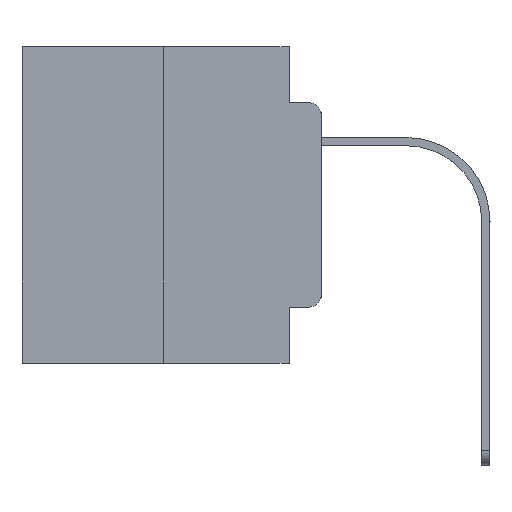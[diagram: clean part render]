
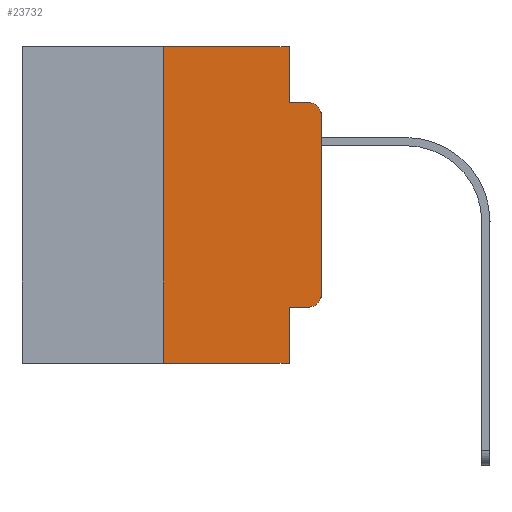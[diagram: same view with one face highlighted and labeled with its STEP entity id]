
A CAD part, left-side view. The second image highlights one B-rep face of the part: STEP entity #23732.
In plain terms, the highlighted planar face has unit normal (-1, 0, 0).
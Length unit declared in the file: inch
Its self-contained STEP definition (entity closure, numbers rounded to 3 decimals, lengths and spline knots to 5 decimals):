
#947 = DIRECTION ( 'NONE',  ( 0., 0., -1. ) ) ;
#1377 = VERTEX_POINT ( 'NONE', #18066 ) ;
#1506 = CARTESIAN_POINT ( 'NONE',  ( 0., 0.25, -0.5 ) ) ;
#1609 = ORIENTED_EDGE ( 'NONE', *, *, #25175, .T. ) ;
#1762 = DIRECTION ( 'NONE',  ( 0., 0., -1. ) ) ;
#2124 = LINE ( 'NONE', #24417, #17803 ) ;
#2192 = EDGE_CURVE ( 'NONE', #19842, #1377, #24350, .T. ) ;
#2422 = EDGE_CURVE ( 'NONE', #10947, #17427, #18857, .T. ) ;
#3428 = EDGE_LOOP ( 'NONE', ( #13011, #10443, #11672, #5072, #9242, #23364, #1609, #8215, #8665, #24004 ) ) ;
#3785 = CARTESIAN_POINT ( 'NONE',  ( 0., 0.02, -0.4115 ) ) ;
#4197 = DIRECTION ( 'NONE',  ( 1., 0., 0. ) ) ;
#4247 = VERTEX_POINT ( 'NONE', #20946 ) ;
#4611 = VERTEX_POINT ( 'NONE', #22001 ) ;
#4989 = EDGE_CURVE ( 'NONE', #5991, #12373, #5500, .T. ) ;
#5072 = ORIENTED_EDGE ( 'NONE', *, *, #4989, .F. ) ;
#5221 = VERTEX_POINT ( 'NONE', #23265 ) ;
#5241 = VECTOR ( 'NONE', #11041, 39.37008 ) ;
#5360 = VECTOR ( 'NONE', #20529, 39.37008 ) ;
#5500 = LINE ( 'NONE', #20105, #22232 ) ;
#5735 = CARTESIAN_POINT ( 'NONE',  ( 0., 0.051, -0.0885 ) ) ;
#5933 = CARTESIAN_POINT ( 'NONE',  ( 0., 0., 0. ) ) ;
#5991 = VERTEX_POINT ( 'NONE', #19231 ) ;
#6164 = DIRECTION ( 'NONE',  ( 0., 0., 1. ) ) ;
#6793 = LINE ( 'NONE', #20867, #22208 ) ;
#7265 = EDGE_CURVE ( 'NONE', #4247, #5991, #6793, .T. ) ;
#7320 = EDGE_CURVE ( 'NONE', #5221, #4611, #13033, .T. ) ;
#8069 = CARTESIAN_POINT ( 'NONE',  ( 0., 0.051, -0.0885 ) ) ;
#8214 = VECTOR ( 'NONE', #14073, 39.37008 ) ;
#8215 = ORIENTED_EDGE ( 'NONE', *, *, #7320, .F. ) ;
#8660 = DIRECTION ( 'NONE',  ( 0., -1., 0. ) ) ;
#8665 = ORIENTED_EDGE ( 'NONE', *, *, #16929, .T. ) ;
#9242 = ORIENTED_EDGE ( 'NONE', *, *, #7265, .F. ) ;
#9701 = VECTOR ( 'NONE', #24666, 39.37008 ) ;
#9929 = AXIS2_PLACEMENT_3D ( 'NONE', #12267, #19970, #1762 ) ;
#10443 = ORIENTED_EDGE ( 'NONE', *, *, #2422, .T. ) ;
#10947 = VERTEX_POINT ( 'NONE', #19371 ) ;
#11041 = DIRECTION ( 'NONE',  ( 0., 0., -1. ) ) ;
#11065 = EDGE_CURVE ( 'NONE', #26241, #4247, #18271, .T. ) ;
#11672 = ORIENTED_EDGE ( 'NONE', *, *, #14029, .F. ) ;
#12267 = CARTESIAN_POINT ( 'NONE',  ( 0., 0.02, -0.3915 ) ) ;
#12313 = DIRECTION ( 'NONE',  ( 0., 0., -1. ) ) ;
#12373 = VERTEX_POINT ( 'NONE', #8069 ) ;
#13011 = ORIENTED_EDGE ( 'NONE', *, *, #23747, .T. ) ;
#13033 = LINE ( 'NONE', #15281, #5241 ) ;
#13389 = VECTOR ( 'NONE', #6164, 39.37008 ) ;
#14029 = EDGE_CURVE ( 'NONE', #12373, #17427, #20067, .T. ) ;
#14073 = DIRECTION ( 'NONE',  ( 0., -1., 0. ) ) ;
#15281 = CARTESIAN_POINT ( 'NONE',  ( 0., 0.051, 0. ) ) ;
#15462 = AXIS2_PLACEMENT_3D ( 'NONE', #23257, #17417, #947 ) ;
#16158 = FACE_OUTER_BOUND ( 'NONE', #3428, .T. ) ;
#16426 = LINE ( 'NONE', #5933, #5360 ) ;
#16591 = CARTESIAN_POINT ( 'NONE',  ( 0., 0.473, -0.5 ) ) ;
#16662 = CARTESIAN_POINT ( 'NONE',  ( 0., 0.25, 0. ) ) ;
#16929 = EDGE_CURVE ( 'NONE', #5221, #19842, #2124, .T. ) ;
#17417 = DIRECTION ( 'NONE',  ( -1., 0., 0. ) ) ;
#17427 = VERTEX_POINT ( 'NONE', #20401 ) ;
#17803 = VECTOR ( 'NONE', #22436, 39.37008 ) ;
#18066 = CARTESIAN_POINT ( 'NONE',  ( 0., 0., -0.3915 ) ) ;
#18271 = LINE ( 'NONE', #16662, #13389 ) ;
#18857 = CIRCLE ( 'NONE', #15462, 0.02 ) ;
#19231 = CARTESIAN_POINT ( 'NONE',  ( 0., 0.051, 0. ) ) ;
#19371 = CARTESIAN_POINT ( 'NONE',  ( 0., 0., -0.1085 ) ) ;
#19842 = VERTEX_POINT ( 'NONE', #3785 ) ;
#19970 = DIRECTION ( 'NONE',  ( -1., 0., 0. ) ) ;
#20067 = LINE ( 'NONE', #5735, #8214 ) ;
#20105 = CARTESIAN_POINT ( 'NONE',  ( 0., 0.051, 0. ) ) ;
#20401 = CARTESIAN_POINT ( 'NONE',  ( 0., 0.02, -0.0885 ) ) ;
#20529 = DIRECTION ( 'NONE',  ( 0., 0., 1. ) ) ;
#20867 = CARTESIAN_POINT ( 'NONE',  ( 0., 0.473, 0. ) ) ;
#20946 = CARTESIAN_POINT ( 'NONE',  ( 0., 0.25, 0. ) ) ;
#20960 = LINE ( 'NONE', #16591, #9701 ) ;
#22001 = CARTESIAN_POINT ( 'NONE',  ( 0., 0.051, -0.5 ) ) ;
#22208 = VECTOR ( 'NONE', #8660, 39.37008 ) ;
#22232 = VECTOR ( 'NONE', #25677, 39.37008 ) ;
#22396 = CARTESIAN_POINT ( 'NONE',  ( 0., 0.473, 0. ) ) ;
#22436 = DIRECTION ( 'NONE',  ( 0., -1., 0. ) ) ;
#23257 = CARTESIAN_POINT ( 'NONE',  ( 0., 0.02, -0.1085 ) ) ;
#23265 = CARTESIAN_POINT ( 'NONE',  ( 0., 0.051, -0.4115 ) ) ;
#23364 = ORIENTED_EDGE ( 'NONE', *, *, #11065, .F. ) ;
#23732 = ADVANCED_FACE ( 'NONE', ( #16158 ), #26250, .F. ) ;
#23747 = EDGE_CURVE ( 'NONE', #1377, #10947, #16426, .T. ) ;
#24004 = ORIENTED_EDGE ( 'NONE', *, *, #2192, .T. ) ;
#24350 = CIRCLE ( 'NONE', #9929, 0.02 ) ;
#24417 = CARTESIAN_POINT ( 'NONE',  ( 0., 0.051, -0.4115 ) ) ;
#24666 = DIRECTION ( 'NONE',  ( 0., -1., 0. ) ) ;
#24865 = AXIS2_PLACEMENT_3D ( 'NONE', #22396, #4197, #12313 ) ;
#25175 = EDGE_CURVE ( 'NONE', #26241, #4611, #20960, .T. ) ;
#25677 = DIRECTION ( 'NONE',  ( 0., 0., -1. ) ) ;
#26241 = VERTEX_POINT ( 'NONE', #1506 ) ;
#26250 = PLANE ( 'NONE',  #24865 ) ;
